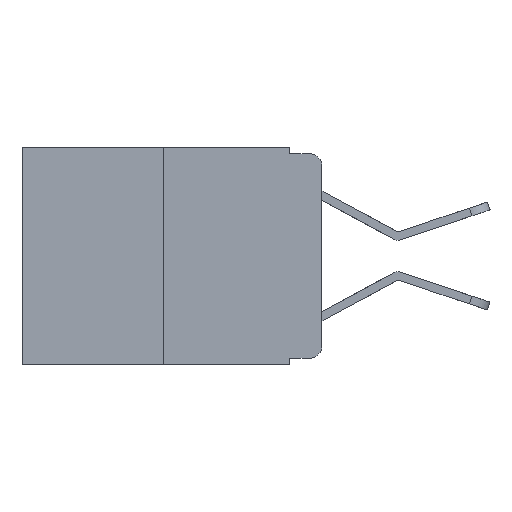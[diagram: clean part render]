
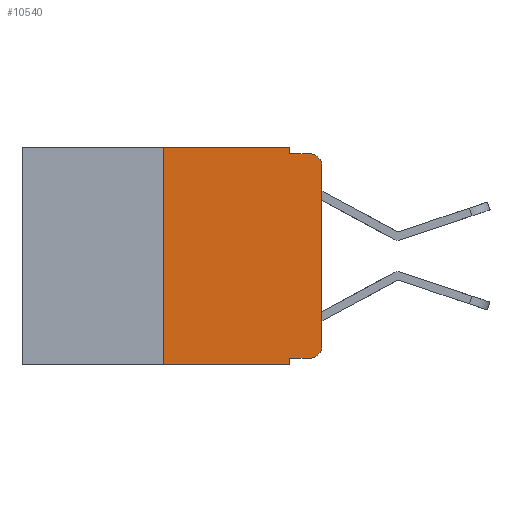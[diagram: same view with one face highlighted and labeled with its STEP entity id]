
A CAD part, left-side view. The second image highlights one B-rep face of the part: STEP entity #10540.
In plain terms, the highlighted planar face has unit normal (-1, 0, 0).
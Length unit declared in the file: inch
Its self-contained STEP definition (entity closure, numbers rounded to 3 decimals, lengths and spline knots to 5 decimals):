
#33 = CARTESIAN_POINT ( 'NONE',  ( 0., 0.473, 0. ) ) ;
#182 = CARTESIAN_POINT ( 'NONE',  ( 0., 0.25, 0. ) ) ;
#183 = DIRECTION ( 'NONE',  ( 0., 0., -1. ) ) ;
#775 = VERTEX_POINT ( 'NONE', #8500 ) ;
#909 = VECTOR ( 'NONE', #5621, 39.37008 ) ;
#973 = DIRECTION ( 'NONE',  ( 0., -1., 0. ) ) ;
#1257 = CARTESIAN_POINT ( 'NONE',  ( 0., 0.051, -0.333 ) ) ;
#1329 = EDGE_CURVE ( 'NONE', #2503, #2738, #9868, .T. ) ;
#1377 = CARTESIAN_POINT ( 'NONE',  ( 0., 0.02, -0.01 ) ) ;
#1468 = VECTOR ( 'NONE', #11089, 39.37008 ) ;
#1597 = ORIENTED_EDGE ( 'NONE', *, *, #2239, .T. ) ;
#1726 = DIRECTION ( 'NONE',  ( 0., -1., 0. ) ) ;
#1745 = LINE ( 'NONE', #9150, #1468 ) ;
#1993 = ORIENTED_EDGE ( 'NONE', *, *, #10016, .F. ) ;
#2058 = CARTESIAN_POINT ( 'NONE',  ( 0., 0.473, -0.343 ) ) ;
#2097 = DIRECTION ( 'NONE',  ( -1., 0., 0. ) ) ;
#2201 = VERTEX_POINT ( 'NONE', #9568 ) ;
#2239 = EDGE_CURVE ( 'NONE', #5627, #7311, #1745, .T. ) ;
#2446 = EDGE_CURVE ( 'NONE', #10523, #7833, #6344, .T. ) ;
#2492 = CARTESIAN_POINT ( 'NONE',  ( 0., 0., -0.313 ) ) ;
#2503 = VERTEX_POINT ( 'NONE', #6297 ) ;
#2520 = DIRECTION ( 'NONE',  ( 0., -1., 0. ) ) ;
#2612 = AXIS2_PLACEMENT_3D ( 'NONE', #5524, #5521, #7180 ) ;
#2738 = VERTEX_POINT ( 'NONE', #5343 ) ;
#3263 = ORIENTED_EDGE ( 'NONE', *, *, #6175, .F. ) ;
#3568 = CARTESIAN_POINT ( 'NONE',  ( 0., 0.051, -0.01 ) ) ;
#3803 = CARTESIAN_POINT ( 'NONE',  ( 0., 0.051, -0.01 ) ) ;
#3853 = CARTESIAN_POINT ( 'NONE',  ( 0., 0.473, 0. ) ) ;
#4121 = ORIENTED_EDGE ( 'NONE', *, *, #7092, .F. ) ;
#4322 = EDGE_CURVE ( 'NONE', #7311, #6081, #7346, .T. ) ;
#4431 = FACE_OUTER_BOUND ( 'NONE', #8627, .T. ) ;
#4724 = LINE ( 'NONE', #33, #11064 ) ;
#5153 = CARTESIAN_POINT ( 'NONE',  ( 0., 0.051, 0. ) ) ;
#5343 = CARTESIAN_POINT ( 'NONE',  ( 0., 0.051, -0.343 ) ) ;
#5463 = VECTOR ( 'NONE', #2520, 39.37008 ) ;
#5521 = DIRECTION ( 'NONE',  ( -1., 0., 0. ) ) ;
#5524 = CARTESIAN_POINT ( 'NONE',  ( 0., 0.02, -0.03 ) ) ;
#5539 = LINE ( 'NONE', #3568, #9673 ) ;
#5557 = AXIS2_PLACEMENT_3D ( 'NONE', #7340, #2097, #8193 ) ;
#5591 = ORIENTED_EDGE ( 'NONE', *, *, #1329, .T. ) ;
#5595 = CARTESIAN_POINT ( 'NONE',  ( 0., 0.051, 0. ) ) ;
#5621 = DIRECTION ( 'NONE',  ( 0., 0., 1. ) ) ;
#5622 = DIRECTION ( 'NONE',  ( 1., 0., 0. ) ) ;
#5627 = VERTEX_POINT ( 'NONE', #2492 ) ;
#5715 = LINE ( 'NONE', #182, #909 ) ;
#5980 = EDGE_CURVE ( 'NONE', #7072, #775, #8346, .T. ) ;
#6000 = DIRECTION ( 'NONE',  ( 0., 0., -1. ) ) ;
#6081 = VERTEX_POINT ( 'NONE', #1377 ) ;
#6175 = EDGE_CURVE ( 'NONE', #7072, #2738, #10911, .T. ) ;
#6297 = CARTESIAN_POINT ( 'NONE',  ( 0., 0.25, -0.343 ) ) ;
#6344 = LINE ( 'NONE', #10310, #10492 ) ;
#6417 = CARTESIAN_POINT ( 'NONE',  ( 0., 0.051, -0.333 ) ) ;
#6514 = DIRECTION ( 'NONE',  ( 0., 0., -1. ) ) ;
#6773 = ORIENTED_EDGE ( 'NONE', *, *, #10082, .F. ) ;
#7072 = VERTEX_POINT ( 'NONE', #6417 ) ;
#7092 = EDGE_CURVE ( 'NONE', #2503, #2201, #5715, .T. ) ;
#7180 = DIRECTION ( 'NONE',  ( 0., 0., -1. ) ) ;
#7311 = VERTEX_POINT ( 'NONE', #11019 ) ;
#7340 = CARTESIAN_POINT ( 'NONE',  ( 0., 0.02, -0.313 ) ) ;
#7346 = CIRCLE ( 'NONE', #2612, 0.02 ) ;
#7833 = VERTEX_POINT ( 'NONE', #3803 ) ;
#7853 = ORIENTED_EDGE ( 'NONE', *, *, #10232, .T. ) ;
#8100 = VECTOR ( 'NONE', #8236, 39.37008 ) ;
#8142 = CIRCLE ( 'NONE', #5557, 0.02 ) ;
#8193 = DIRECTION ( 'NONE',  ( 0., 0., -1. ) ) ;
#8236 = DIRECTION ( 'NONE',  ( 0., -1., 0. ) ) ;
#8346 = LINE ( 'NONE', #1257, #8100 ) ;
#8500 = CARTESIAN_POINT ( 'NONE',  ( 0., 0.02, -0.333 ) ) ;
#8627 = EDGE_LOOP ( 'NONE', ( #1597, #10466, #1993, #11112, #6773, #4121, #5591, #3263, #9307, #7853 ) ) ;
#8676 = AXIS2_PLACEMENT_3D ( 'NONE', #3853, #5622, #183 ) ;
#8727 = VECTOR ( 'NONE', #6000, 39.37008 ) ;
#8926 = PLANE ( 'NONE',  #8676 ) ;
#9150 = CARTESIAN_POINT ( 'NONE',  ( 0., 0., 0. ) ) ;
#9307 = ORIENTED_EDGE ( 'NONE', *, *, #5980, .T. ) ;
#9568 = CARTESIAN_POINT ( 'NONE',  ( 0., 0.25, 0. ) ) ;
#9673 = VECTOR ( 'NONE', #1726, 39.37008 ) ;
#9868 = LINE ( 'NONE', #2058, #5463 ) ;
#10016 = EDGE_CURVE ( 'NONE', #7833, #6081, #5539, .T. ) ;
#10082 = EDGE_CURVE ( 'NONE', #2201, #10523, #4724, .T. ) ;
#10232 = EDGE_CURVE ( 'NONE', #775, #5627, #8142, .T. ) ;
#10310 = CARTESIAN_POINT ( 'NONE',  ( 0., 0.051, 0. ) ) ;
#10466 = ORIENTED_EDGE ( 'NONE', *, *, #4322, .T. ) ;
#10492 = VECTOR ( 'NONE', #6514, 39.37008 ) ;
#10523 = VERTEX_POINT ( 'NONE', #5595 ) ;
#10540 = ADVANCED_FACE ( 'NONE', ( #4431 ), #8926, .F. ) ;
#10911 = LINE ( 'NONE', #5153, #8727 ) ;
#11019 = CARTESIAN_POINT ( 'NONE',  ( 0., 0., -0.03 ) ) ;
#11064 = VECTOR ( 'NONE', #973, 39.37008 ) ;
#11089 = DIRECTION ( 'NONE',  ( 0., 0., 1. ) ) ;
#11112 = ORIENTED_EDGE ( 'NONE', *, *, #2446, .F. ) ;
